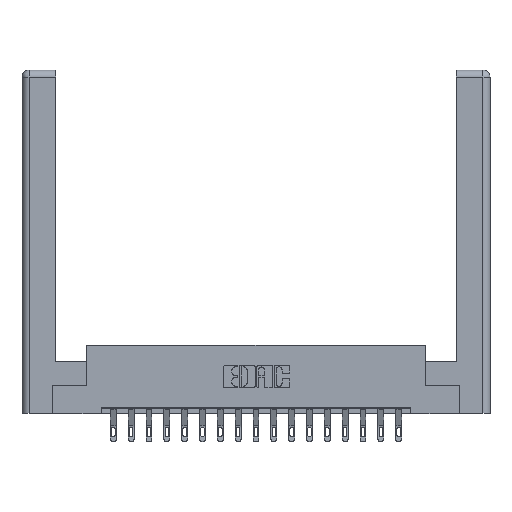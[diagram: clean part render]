
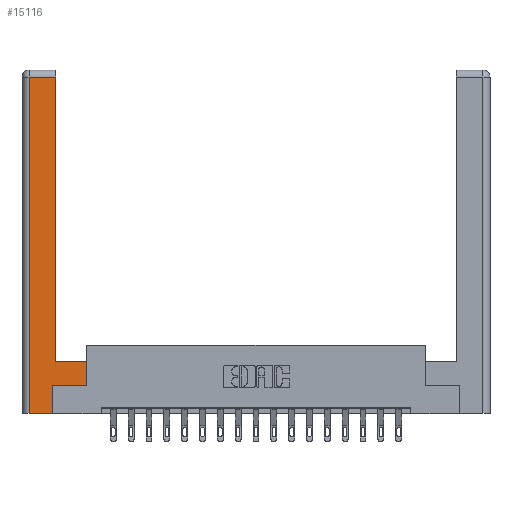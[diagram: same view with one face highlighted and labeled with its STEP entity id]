
A CAD part, top view. The second image highlights one B-rep face of the part: STEP entity #15116.
In plain terms, the highlighted planar face has unit normal (0, 0, 1).
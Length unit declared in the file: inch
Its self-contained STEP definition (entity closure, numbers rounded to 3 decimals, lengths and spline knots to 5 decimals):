
#37 = CARTESIAN_POINT ( 'NONE',  ( 0., 0., 0. ) ) ;
#78 = LINE ( 'NONE', #2636, #14584 ) ;
#373 = CARTESIAN_POINT ( 'NONE',  ( 0.565, 0.245, 0. ) ) ;
#737 = VECTOR ( 'NONE', #14983, 39.37008 ) ;
#1233 = AXIS2_PLACEMENT_3D ( 'NONE', #37, #3245, #13698 ) ;
#1702 = CARTESIAN_POINT ( 'NONE',  ( 0.265, 0.245, 0. ) ) ;
#1889 = LINE ( 'NONE', #1702, #737 ) ;
#1933 = ORIENTED_EDGE ( 'NONE', *, *, #7190, .T. ) ;
#2229 = LINE ( 'NONE', #6811, #16206 ) ;
#2310 = VECTOR ( 'NONE', #7143, 39.37008 ) ;
#2362 = EDGE_CURVE ( 'NONE', #17455, #9643, #13531, .T. ) ;
#2596 = ORIENTED_EDGE ( 'NONE', *, *, #2362, .T. ) ;
#2636 = CARTESIAN_POINT ( 'NONE',  ( 0.0615, 2.94, 0. ) ) ;
#3245 = DIRECTION ( 'NONE',  ( 0., 0., -1. ) ) ;
#4112 = EDGE_LOOP ( 'NONE', ( #19277, #8631, #2596, #1933, #17767, #13298, #14487, #18369 ) ) ;
#4131 = CARTESIAN_POINT ( 'NONE',  ( 0.0615, 0., 0. ) ) ;
#4457 = VECTOR ( 'NONE', #11543, 39.37008 ) ;
#4827 = VECTOR ( 'NONE', #13153, 39.37008 ) ;
#5478 = CARTESIAN_POINT ( 'NONE',  ( 0.295, 0.45, 0. ) ) ;
#5652 = DIRECTION ( 'NONE',  ( -1., 0., 0. ) ) ;
#5938 = CARTESIAN_POINT ( 'NONE',  ( 0.295, 0.45, 0. ) ) ;
#6652 = LINE ( 'NONE', #373, #17166 ) ;
#6811 = CARTESIAN_POINT ( 'NONE',  ( 0.265, 0., 0. ) ) ;
#7143 = DIRECTION ( 'NONE',  ( 0., -1., 0. ) ) ;
#7190 = EDGE_CURVE ( 'NONE', #9643, #17116, #2229, .T. ) ;
#7625 = VERTEX_POINT ( 'NONE', #14975 ) ;
#7988 = LINE ( 'NONE', #18141, #15465 ) ;
#8430 = LINE ( 'NONE', #5478, #4457 ) ;
#8631 = ORIENTED_EDGE ( 'NONE', *, *, #19387, .T. ) ;
#9244 = DIRECTION ( 'NONE',  ( 0., 1., 0. ) ) ;
#9583 = VERTEX_POINT ( 'NONE', #5938 ) ;
#9643 = VERTEX_POINT ( 'NONE', #13521 ) ;
#9737 = CARTESIAN_POINT ( 'NONE',  ( 0.265, 0.245, 0. ) ) ;
#9903 = EDGE_CURVE ( 'NONE', #9583, #17403, #7988, .T. ) ;
#10018 = EDGE_CURVE ( 'NONE', #7625, #9583, #8430, .T. ) ;
#11173 = DIRECTION ( 'NONE',  ( 1., 0., 0. ) ) ;
#11543 = DIRECTION ( 'NONE',  ( -1., 0., 0. ) ) ;
#13153 = DIRECTION ( 'NONE',  ( 0., 1., 0. ) ) ;
#13298 = ORIENTED_EDGE ( 'NONE', *, *, #18493, .T. ) ;
#13485 = EDGE_CURVE ( 'NONE', #17116, #14967, #1889, .T. ) ;
#13521 = CARTESIAN_POINT ( 'NONE',  ( 0.0615, 0., 0. ) ) ;
#13531 = LINE ( 'NONE', #4131, #2310 ) ;
#13698 = DIRECTION ( 'NONE',  ( -1., 0., 0. ) ) ;
#13702 = LINE ( 'NONE', #14716, #4827 ) ;
#13762 = PLANE ( 'NONE',  #1233 ) ;
#14487 = ORIENTED_EDGE ( 'NONE', *, *, #16155, .T. ) ;
#14584 = VECTOR ( 'NONE', #5652, 39.37008 ) ;
#14716 = CARTESIAN_POINT ( 'NONE',  ( 0.565, 0.45, 0. ) ) ;
#14967 = VERTEX_POINT ( 'NONE', #9737 ) ;
#14975 = CARTESIAN_POINT ( 'NONE',  ( 0.565, 0.45, 0. ) ) ;
#14983 = DIRECTION ( 'NONE',  ( 0., 1., 0. ) ) ;
#15116 = ADVANCED_FACE ( 'NONE', ( #18702 ), #13762, .F. ) ;
#15168 = VERTEX_POINT ( 'NONE', #16410 ) ;
#15465 = VECTOR ( 'NONE', #9244, 39.37008 ) ;
#15852 = CARTESIAN_POINT ( 'NONE',  ( 0.0615, 2.94, 0. ) ) ;
#16155 = EDGE_CURVE ( 'NONE', #15168, #7625, #13702, .T. ) ;
#16206 = VECTOR ( 'NONE', #18773, 39.37008 ) ;
#16410 = CARTESIAN_POINT ( 'NONE',  ( 0.565, 0.245, 0. ) ) ;
#17116 = VERTEX_POINT ( 'NONE', #17505 ) ;
#17166 = VECTOR ( 'NONE', #11173, 39.37008 ) ;
#17375 = CARTESIAN_POINT ( 'NONE',  ( 0.295, 2.94, 0. ) ) ;
#17403 = VERTEX_POINT ( 'NONE', #17375 ) ;
#17455 = VERTEX_POINT ( 'NONE', #15852 ) ;
#17505 = CARTESIAN_POINT ( 'NONE',  ( 0.265, 0., 0. ) ) ;
#17767 = ORIENTED_EDGE ( 'NONE', *, *, #13485, .T. ) ;
#18141 = CARTESIAN_POINT ( 'NONE',  ( 0.295, 3., 0. ) ) ;
#18369 = ORIENTED_EDGE ( 'NONE', *, *, #10018, .T. ) ;
#18493 = EDGE_CURVE ( 'NONE', #14967, #15168, #6652, .T. ) ;
#18702 = FACE_OUTER_BOUND ( 'NONE', #4112, .T. ) ;
#18773 = DIRECTION ( 'NONE',  ( 1., 0., 0. ) ) ;
#19277 = ORIENTED_EDGE ( 'NONE', *, *, #9903, .T. ) ;
#19387 = EDGE_CURVE ( 'NONE', #17403, #17455, #78, .T. ) ;
